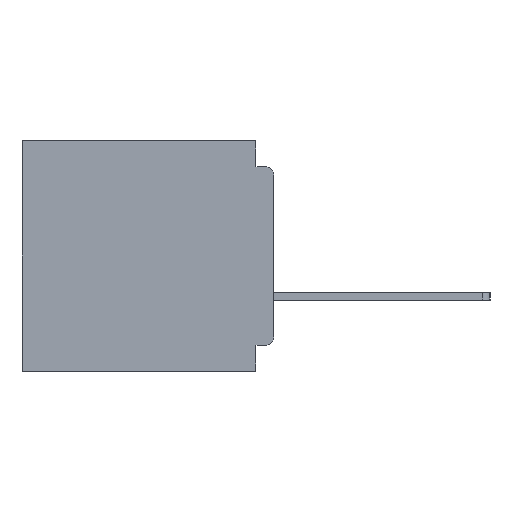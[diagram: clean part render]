
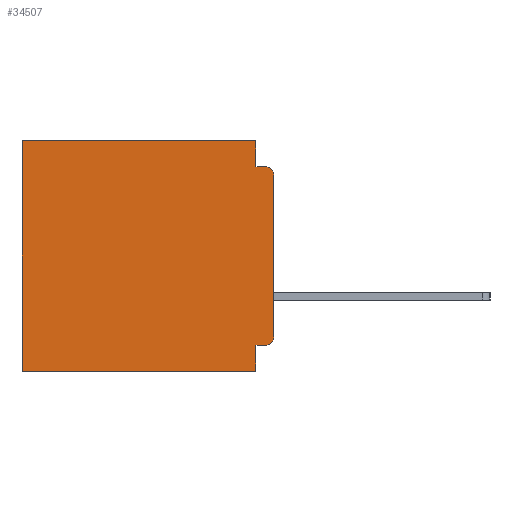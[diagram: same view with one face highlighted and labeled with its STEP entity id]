
A CAD part, left-side view. The second image highlights one B-rep face of the part: STEP entity #34507.
In plain terms, the highlighted planar face has unit normal (-1, 0, 0).
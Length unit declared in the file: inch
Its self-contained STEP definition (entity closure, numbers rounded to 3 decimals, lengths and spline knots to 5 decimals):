
#267 = VERTEX_POINT ( 'NONE', #24861 ) ;
#447 = DIRECTION ( 'NONE',  ( 0., 0., -1. ) ) ;
#565 = DIRECTION ( 'NONE',  ( -1., 0., 0. ) ) ;
#577 = CARTESIAN_POINT ( 'NONE',  ( 0.3, 0.015, -0.34 ) ) ;
#1142 = PLANE ( 'NONE',  #14495 ) ;
#1640 = ORIENTED_EDGE ( 'NONE', *, *, #20024, .F. ) ;
#1753 = EDGE_CURVE ( 'NONE', #23934, #1863, #23862, .T. ) ;
#1863 = VERTEX_POINT ( 'NONE', #25711 ) ;
#2456 = VECTOR ( 'NONE', #17391, 39.37008 ) ;
#2917 = LINE ( 'NONE', #23240, #30506 ) ;
#3541 = VERTEX_POINT ( 'NONE', #7696 ) ;
#4172 = EDGE_CURVE ( 'NONE', #3541, #267, #34007, .T. ) ;
#5031 = LINE ( 'NONE', #13344, #25530 ) ;
#5398 = LINE ( 'NONE', #5911, #25910 ) ;
#5911 = CARTESIAN_POINT ( 'NONE',  ( 0.3, 0., -0.355 ) ) ;
#5941 = ORIENTED_EDGE ( 'NONE', *, *, #23580, .F. ) ;
#6049 = VECTOR ( 'NONE', #13292, 39.37008 ) ;
#6382 = ORIENTED_EDGE ( 'NONE', *, *, #4172, .F. ) ;
#6477 = CIRCLE ( 'NONE', #33357, 0.015 ) ;
#7146 = CARTESIAN_POINT ( 'NONE',  ( 0.3, 0.031, 0. ) ) ;
#7198 = CARTESIAN_POINT ( 'NONE',  ( 0.3, 0.015, -0.06 ) ) ;
#7696 = CARTESIAN_POINT ( 'NONE',  ( 0.3, 0.031, -0.045 ) ) ;
#8053 = CARTESIAN_POINT ( 'NONE',  ( 0.3, 0.031, -0.355 ) ) ;
#8543 = FACE_OUTER_BOUND ( 'NONE', #25647, .T. ) ;
#8837 = ORIENTED_EDGE ( 'NONE', *, *, #14448, .F. ) ;
#9549 = LINE ( 'NONE', #7146, #22963 ) ;
#9836 = DIRECTION ( 'NONE',  ( 0., 0., -1. ) ) ;
#9889 = DIRECTION ( 'NONE',  ( 0., 0., -1. ) ) ;
#10463 = AXIS2_PLACEMENT_3D ( 'NONE', #577, #565, #447 ) ;
#10944 = CARTESIAN_POINT ( 'NONE',  ( 0.3, 0., -0.06 ) ) ;
#11447 = EDGE_CURVE ( 'NONE', #13272, #27776, #23962, .T. ) ;
#12605 = DIRECTION ( 'NONE',  ( 0., 0., -1. ) ) ;
#12886 = VECTOR ( 'NONE', #20462, 39.37008 ) ;
#13153 = LINE ( 'NONE', #29244, #6049 ) ;
#13272 = VERTEX_POINT ( 'NONE', #32087 ) ;
#13292 = DIRECTION ( 'NONE',  ( 0., 0., -1. ) ) ;
#13344 = CARTESIAN_POINT ( 'NONE',  ( 0.3, 0., -0.4 ) ) ;
#13799 = DIRECTION ( 'NONE',  ( 0., 0., -1. ) ) ;
#14448 = EDGE_CURVE ( 'NONE', #18704, #25445, #5031, .T. ) ;
#14495 = AXIS2_PLACEMENT_3D ( 'NONE', #27883, #30614, #14711 ) ;
#14711 = DIRECTION ( 'NONE',  ( 0., 0., -1. ) ) ;
#14935 = CARTESIAN_POINT ( 'NONE',  ( 0.3, 0., 0. ) ) ;
#15511 = CARTESIAN_POINT ( 'NONE',  ( 0.3, 0.437, -0.4 ) ) ;
#16055 = DIRECTION ( 'NONE',  ( 0., 1., 0. ) ) ;
#16946 = CARTESIAN_POINT ( 'NONE',  ( 0.3, 0., -0.34 ) ) ;
#17391 = DIRECTION ( 'NONE',  ( 0., 1., 0. ) ) ;
#18704 = VERTEX_POINT ( 'NONE', #27795 ) ;
#20024 = EDGE_CURVE ( 'NONE', #24280, #18704, #22812, .T. ) ;
#20389 = EDGE_CURVE ( 'NONE', #30315, #267, #6477, .T. ) ;
#20462 = DIRECTION ( 'NONE',  ( 0., -1., 0. ) ) ;
#20560 = EDGE_CURVE ( 'NONE', #30315, #27776, #13153, .T. ) ;
#20994 = ORIENTED_EDGE ( 'NONE', *, *, #20560, .F. ) ;
#21393 = ORIENTED_EDGE ( 'NONE', *, *, #22131, .T. ) ;
#22131 = EDGE_CURVE ( 'NONE', #1863, #25445, #2917, .T. ) ;
#22812 = LINE ( 'NONE', #27102, #29843 ) ;
#22963 = VECTOR ( 'NONE', #9836, 39.37008 ) ;
#23069 = ORIENTED_EDGE ( 'NONE', *, *, #23297, .F. ) ;
#23240 = CARTESIAN_POINT ( 'NONE',  ( 0.3, 0.437, -0.4 ) ) ;
#23297 = EDGE_CURVE ( 'NONE', #13272, #24280, #5398, .T. ) ;
#23580 = EDGE_CURVE ( 'NONE', #23934, #3541, #9549, .T. ) ;
#23862 = LINE ( 'NONE', #14935, #2456 ) ;
#23934 = VERTEX_POINT ( 'NONE', #32837 ) ;
#23962 = CIRCLE ( 'NONE', #10463, 0.015 ) ;
#24280 = VERTEX_POINT ( 'NONE', #8053 ) ;
#24861 = CARTESIAN_POINT ( 'NONE',  ( 0.3, 0.015, -0.045 ) ) ;
#25445 = VERTEX_POINT ( 'NONE', #15511 ) ;
#25530 = VECTOR ( 'NONE', #16055, 39.37008 ) ;
#25647 = EDGE_LOOP ( 'NONE', ( #20994, #26846, #6382, #5941, #34170, #21393, #8837, #1640, #23069, #30529 ) ) ;
#25711 = CARTESIAN_POINT ( 'NONE',  ( 0.3, 0.437, 0. ) ) ;
#25910 = VECTOR ( 'NONE', #32521, 39.37008 ) ;
#25927 = DIRECTION ( 'NONE',  ( -1., 0., 0. ) ) ;
#26846 = ORIENTED_EDGE ( 'NONE', *, *, #20389, .T. ) ;
#27102 = CARTESIAN_POINT ( 'NONE',  ( 0.3, 0.031, -0.4 ) ) ;
#27562 = CARTESIAN_POINT ( 'NONE',  ( 0.3, 0., -0.045 ) ) ;
#27776 = VERTEX_POINT ( 'NONE', #16946 ) ;
#27795 = CARTESIAN_POINT ( 'NONE',  ( 0.3, 0.031, -0.4 ) ) ;
#27883 = CARTESIAN_POINT ( 'NONE',  ( 0.3, 0., -0.4 ) ) ;
#29244 = CARTESIAN_POINT ( 'NONE',  ( 0.3, 0., -0.4 ) ) ;
#29843 = VECTOR ( 'NONE', #13799, 39.37008 ) ;
#30315 = VERTEX_POINT ( 'NONE', #10944 ) ;
#30506 = VECTOR ( 'NONE', #12605, 39.37008 ) ;
#30529 = ORIENTED_EDGE ( 'NONE', *, *, #11447, .T. ) ;
#30614 = DIRECTION ( 'NONE',  ( 1., 0., 0. ) ) ;
#32087 = CARTESIAN_POINT ( 'NONE',  ( 0.3, 0.015, -0.355 ) ) ;
#32521 = DIRECTION ( 'NONE',  ( 0., 1., 0. ) ) ;
#32837 = CARTESIAN_POINT ( 'NONE',  ( 0.3, 0.031, 0. ) ) ;
#33357 = AXIS2_PLACEMENT_3D ( 'NONE', #7198, #25927, #9889 ) ;
#34007 = LINE ( 'NONE', #27562, #12886 ) ;
#34170 = ORIENTED_EDGE ( 'NONE', *, *, #1753, .T. ) ;
#34507 = ADVANCED_FACE ( 'NONE', ( #8543 ), #1142, .F. ) ;
